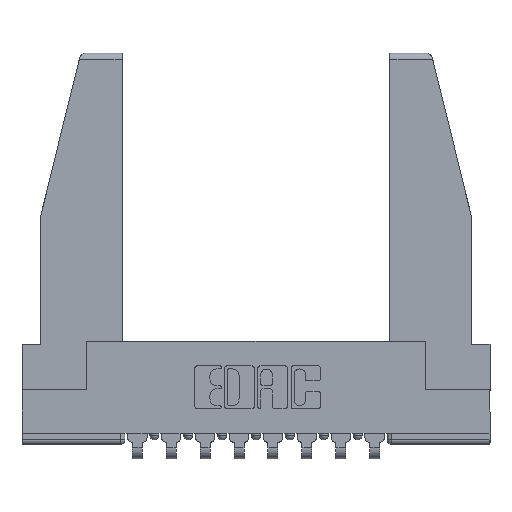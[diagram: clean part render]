
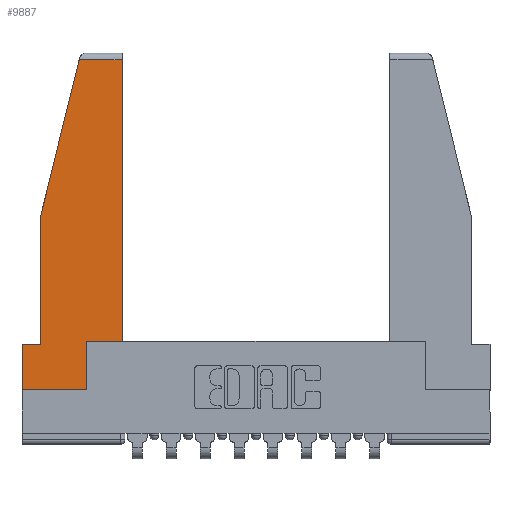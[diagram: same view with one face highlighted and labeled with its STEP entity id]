
A CAD part, top view. The second image highlights one B-rep face of the part: STEP entity #9887.
In plain terms, the highlighted planar face has unit normal (0, 0, 1).
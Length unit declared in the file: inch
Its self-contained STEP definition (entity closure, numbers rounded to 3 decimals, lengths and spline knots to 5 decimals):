
#129 = CARTESIAN_POINT ( 'NONE',  ( 0.297, 0., 0. ) ) ;
#210 = LINE ( 'NONE', #8292, #12099 ) ;
#339 = VERTEX_POINT ( 'NONE', #4747 ) ;
#341 = EDGE_CURVE ( 'NONE', #703, #3537, #6747, .T. ) ;
#542 = DIRECTION ( 'NONE',  ( 0., -1., 0. ) ) ;
#703 = VERTEX_POINT ( 'NONE', #5014 ) ;
#756 = VECTOR ( 'NONE', #11906, 39.37008 ) ;
#1200 = ORIENTED_EDGE ( 'NONE', *, *, #4814, .T. ) ;
#1369 = CARTESIAN_POINT ( 'NONE',  ( 0., 0.21, 0. ) ) ;
#1378 = VECTOR ( 'NONE', #542, 39.37008 ) ;
#1847 = ORIENTED_EDGE ( 'NONE', *, *, #5596, .T. ) ;
#2400 = VECTOR ( 'NONE', #12855, 39.37008 ) ;
#2495 = ORIENTED_EDGE ( 'NONE', *, *, #10496, .T. ) ;
#2511 = DIRECTION ( 'NONE',  ( 0., 0., 1. ) ) ;
#2578 = CARTESIAN_POINT ( 'NONE',  ( 0., 0., 0. ) ) ;
#2657 = EDGE_CURVE ( 'NONE', #11837, #8510, #2986, .T. ) ;
#2986 = LINE ( 'NONE', #11653, #4710 ) ;
#3027 = ORIENTED_EDGE ( 'NONE', *, *, #2657, .T. ) ;
#3534 = CARTESIAN_POINT ( 'NONE',  ( 0.297, 0.223, 0. ) ) ;
#3537 = VERTEX_POINT ( 'NONE', #11882 ) ;
#3596 = AXIS2_PLACEMENT_3D ( 'NONE', #2578, #2511, #8872 ) ;
#3624 = PLANE ( 'NONE',  #3596 ) ;
#4108 = ORIENTED_EDGE ( 'NONE', *, *, #5206, .T. ) ;
#4329 = LINE ( 'NONE', #1369, #756 ) ;
#4432 = ORIENTED_EDGE ( 'NONE', *, *, #341, .T. ) ;
#4710 = VECTOR ( 'NONE', #7178, 39.37008 ) ;
#4725 = DIRECTION ( 'NONE',  ( 0., 1., 0. ) ) ;
#4747 = CARTESIAN_POINT ( 'NONE',  ( 0.086, 0.8, 0. ) ) ;
#4771 = EDGE_CURVE ( 'NONE', #3537, #10768, #13483, .T. ) ;
#4814 = EDGE_CURVE ( 'NONE', #8510, #9172, #10774, .T. ) ;
#4833 = VECTOR ( 'NONE', #6883, 39.37008 ) ;
#4965 = VERTEX_POINT ( 'NONE', #10290 ) ;
#5014 = CARTESIAN_POINT ( 'NONE',  ( 0., 0.21, 0. ) ) ;
#5206 = EDGE_CURVE ( 'NONE', #4965, #339, #210, .T. ) ;
#5312 = DIRECTION ( 'NONE',  ( -0.239, -0.971, 0. ) ) ;
#5494 = CARTESIAN_POINT ( 'NONE',  ( 0.297, 0., 0. ) ) ;
#5596 = EDGE_CURVE ( 'NONE', #10768, #11837, #6333, .T. ) ;
#5763 = ORIENTED_EDGE ( 'NONE', *, *, #4771, .T. ) ;
#5803 = VECTOR ( 'NONE', #9739, 39.37008 ) ;
#6333 = LINE ( 'NONE', #129, #7447 ) ;
#6566 = EDGE_CURVE ( 'NONE', #339, #8737, #9090, .T. ) ;
#6651 = CARTESIAN_POINT ( 'NONE',  ( 0.086, 0.21, 0. ) ) ;
#6747 = LINE ( 'NONE', #12177, #1378 ) ;
#6748 = CARTESIAN_POINT ( 'NONE',  ( 0.086, 0.8, 0. ) ) ;
#6883 = DIRECTION ( 'NONE',  ( 0., -1., 0. ) ) ;
#6900 = ORIENTED_EDGE ( 'NONE', *, *, #12613, .T. ) ;
#7028 = VECTOR ( 'NONE', #4725, 39.37008 ) ;
#7178 = DIRECTION ( 'NONE',  ( 1., 0., 0. ) ) ;
#7447 = VECTOR ( 'NONE', #10478, 39.37008 ) ;
#7465 = CARTESIAN_POINT ( 'NONE',  ( 0.461, 0.223, 0. ) ) ;
#7785 = ORIENTED_EDGE ( 'NONE', *, *, #6566, .T. ) ;
#7818 = CARTESIAN_POINT ( 'NONE',  ( 0.461, 0.223, 0. ) ) ;
#8177 = CARTESIAN_POINT ( 'NONE',  ( 0.461, 1.52, 0. ) ) ;
#8292 = CARTESIAN_POINT ( 'NONE',  ( 0.271, 1.55, 0. ) ) ;
#8510 = VERTEX_POINT ( 'NONE', #7465 ) ;
#8655 = CARTESIAN_POINT ( 'NONE',  ( 0., 0., 0. ) ) ;
#8737 = VERTEX_POINT ( 'NONE', #6651 ) ;
#8872 = DIRECTION ( 'NONE',  ( 1., 0., 0. ) ) ;
#9090 = LINE ( 'NONE', #6748, #4833 ) ;
#9172 = VERTEX_POINT ( 'NONE', #8177 ) ;
#9175 = EDGE_LOOP ( 'NONE', ( #1200, #2495, #4108, #7785, #6900, #4432, #5763, #1847, #3027 ) ) ;
#9739 = DIRECTION ( 'NONE',  ( -1., 0., 0. ) ) ;
#9887 = ADVANCED_FACE ( 'NONE', ( #11679 ), #3624, .T. ) ;
#10290 = CARTESIAN_POINT ( 'NONE',  ( 0.2636, 1.52, 0. ) ) ;
#10478 = DIRECTION ( 'NONE',  ( 0., 1., 0. ) ) ;
#10496 = EDGE_CURVE ( 'NONE', #9172, #4965, #10692, .T. ) ;
#10692 = LINE ( 'NONE', #11729, #5803 ) ;
#10768 = VERTEX_POINT ( 'NONE', #5494 ) ;
#10774 = LINE ( 'NONE', #7818, #7028 ) ;
#11653 = CARTESIAN_POINT ( 'NONE',  ( 0.297, 0.223, 0. ) ) ;
#11679 = FACE_OUTER_BOUND ( 'NONE', #9175, .T. ) ;
#11729 = CARTESIAN_POINT ( 'NONE',  ( 0., 1.52, 0. ) ) ;
#11837 = VERTEX_POINT ( 'NONE', #3534 ) ;
#11882 = CARTESIAN_POINT ( 'NONE',  ( 0., 0., 0. ) ) ;
#11906 = DIRECTION ( 'NONE',  ( -1., 0., 0. ) ) ;
#12099 = VECTOR ( 'NONE', #5312, 39.37008 ) ;
#12177 = CARTESIAN_POINT ( 'NONE',  ( 0., 0.21, 0. ) ) ;
#12613 = EDGE_CURVE ( 'NONE', #8737, #703, #4329, .T. ) ;
#12855 = DIRECTION ( 'NONE',  ( 1., 0., 0. ) ) ;
#13483 = LINE ( 'NONE', #8655, #2400 ) ;
